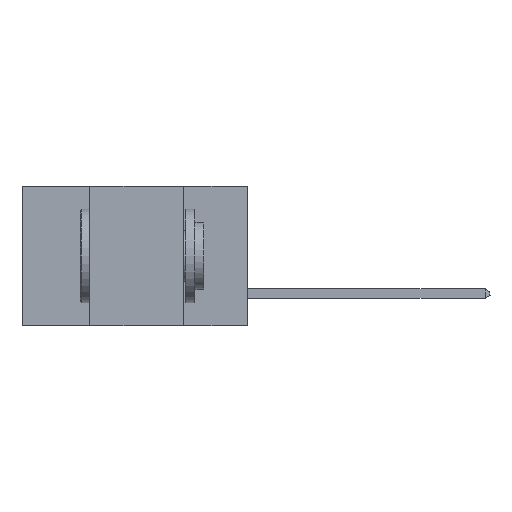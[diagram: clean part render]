
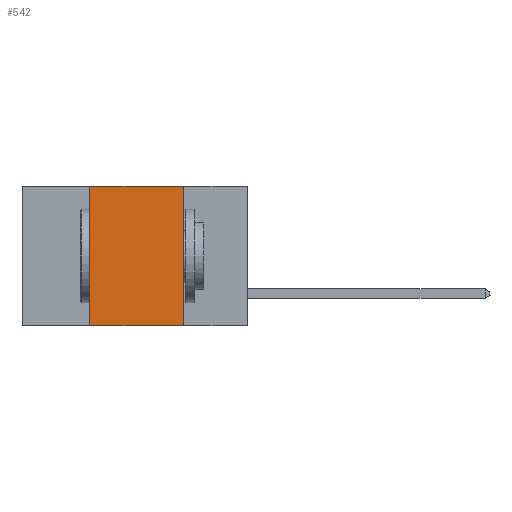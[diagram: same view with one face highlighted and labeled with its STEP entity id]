
A CAD part, left-side view. The second image highlights one B-rep face of the part: STEP entity #542.
In plain terms, the highlighted planar face has unit normal (-1, 0, 0).
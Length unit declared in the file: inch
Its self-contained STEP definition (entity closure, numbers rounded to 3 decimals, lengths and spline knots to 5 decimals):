
#190 = EDGE_CURVE ( 'NONE', #4734, #12712, #12938, .T. ) ;
#428 = LINE ( 'NONE', #1262, #5184 ) ;
#542 = ADVANCED_FACE ( 'NONE', ( #7519 ), #5101, .F. ) ;
#1084 = VERTEX_POINT ( 'NONE', #10943 ) ;
#1262 = CARTESIAN_POINT ( 'NONE',  ( 0., 0.6, 0. ) ) ;
#1731 = DIRECTION ( 'NONE',  ( 0., 0., -1. ) ) ;
#2257 = CARTESIAN_POINT ( 'NONE',  ( 0., 0.17, 0. ) ) ;
#2593 = ORIENTED_EDGE ( 'NONE', *, *, #6197, .F. ) ;
#2942 = VECTOR ( 'NONE', #5942, 39.37008 ) ;
#4060 = EDGE_CURVE ( 'NONE', #13408, #12712, #4087, .T. ) ;
#4087 = LINE ( 'NONE', #11138, #10187 ) ;
#4734 = VERTEX_POINT ( 'NONE', #9121 ) ;
#5074 = ORIENTED_EDGE ( 'NONE', *, *, #8076, .F. ) ;
#5101 = PLANE ( 'NONE',  #5455 ) ;
#5184 = VECTOR ( 'NONE', #11781, 39.37008 ) ;
#5455 = AXIS2_PLACEMENT_3D ( 'NONE', #12444, #10393, #6145 ) ;
#5942 = DIRECTION ( 'NONE',  ( 0., 0., 1. ) ) ;
#6145 = DIRECTION ( 'NONE',  ( 0., 0., -1. ) ) ;
#6197 = EDGE_CURVE ( 'NONE', #4734, #1084, #8867, .T. ) ;
#7519 = FACE_OUTER_BOUND ( 'NONE', #8780, .T. ) ;
#7693 = VECTOR ( 'NONE', #13144, 39.37008 ) ;
#8076 = EDGE_CURVE ( 'NONE', #1084, #13408, #428, .T. ) ;
#8609 = CARTESIAN_POINT ( 'NONE',  ( 0., 0.17, -0.37 ) ) ;
#8780 = EDGE_LOOP ( 'NONE', ( #11113, #5074, #2593, #13289 ) ) ;
#8867 = LINE ( 'NONE', #9141, #2942 ) ;
#9030 = CARTESIAN_POINT ( 'NONE',  ( 0., 0.6, -0.37 ) ) ;
#9121 = CARTESIAN_POINT ( 'NONE',  ( 0., 0.42, -0.37 ) ) ;
#9141 = CARTESIAN_POINT ( 'NONE',  ( 0., 0.42, 0. ) ) ;
#10187 = VECTOR ( 'NONE', #1731, 39.37008 ) ;
#10393 = DIRECTION ( 'NONE',  ( 1., 0., 0. ) ) ;
#10943 = CARTESIAN_POINT ( 'NONE',  ( 0., 0.42, 0. ) ) ;
#11113 = ORIENTED_EDGE ( 'NONE', *, *, #4060, .F. ) ;
#11138 = CARTESIAN_POINT ( 'NONE',  ( 0., 0.17, 0. ) ) ;
#11781 = DIRECTION ( 'NONE',  ( 0., -1., 0. ) ) ;
#12444 = CARTESIAN_POINT ( 'NONE',  ( 0., 0.6, 0. ) ) ;
#12712 = VERTEX_POINT ( 'NONE', #8609 ) ;
#12938 = LINE ( 'NONE', #9030, #7693 ) ;
#13144 = DIRECTION ( 'NONE',  ( 0., -1., 0. ) ) ;
#13289 = ORIENTED_EDGE ( 'NONE', *, *, #190, .T. ) ;
#13408 = VERTEX_POINT ( 'NONE', #2257 ) ;
